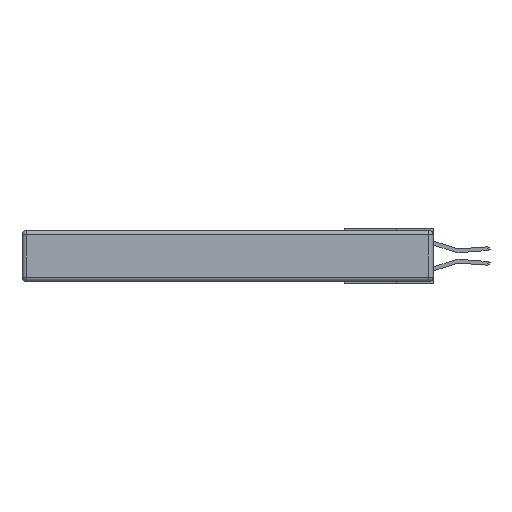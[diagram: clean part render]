
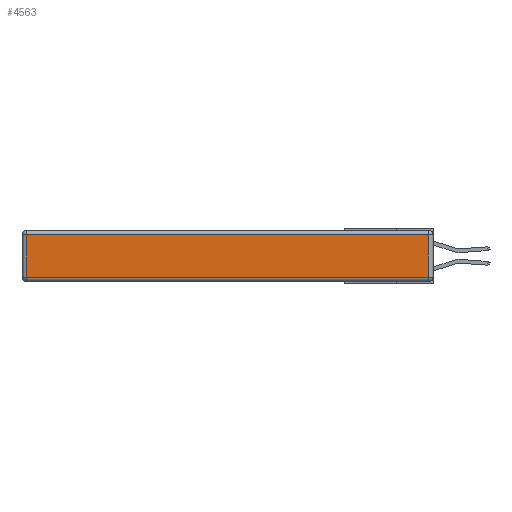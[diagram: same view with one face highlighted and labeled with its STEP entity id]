
A CAD part, left-side view. The second image highlights one B-rep face of the part: STEP entity #4563.
In plain terms, the highlighted planar face has unit normal (-1, 0, 0).
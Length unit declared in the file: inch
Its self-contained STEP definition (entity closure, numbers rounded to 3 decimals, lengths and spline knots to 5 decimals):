
#254 = EDGE_LOOP ( 'NONE', ( #12194, #11141, #3514, #7968 ) ) ;
#771 = CARTESIAN_POINT ( 'NONE',  ( 0., 0.03, -0.313 ) ) ;
#795 = VERTEX_POINT ( 'NONE', #9223 ) ;
#1589 = VECTOR ( 'NONE', #9602, 39.37008 ) ;
#1699 = DIRECTION ( 'NONE',  ( 0., 0., 1. ) ) ;
#2094 = VECTOR ( 'NONE', #2577, 39.37008 ) ;
#2219 = DIRECTION ( 'NONE',  ( 0., 0., 1. ) ) ;
#2357 = EDGE_CURVE ( 'NONE', #6201, #795, #15853, .T. ) ;
#2577 = DIRECTION ( 'NONE',  ( 0., -1., 0. ) ) ;
#3514 = ORIENTED_EDGE ( 'NONE', *, *, #5901, .T. ) ;
#4123 = CARTESIAN_POINT ( 'NONE',  ( 0., 0.03, -0.343 ) ) ;
#4563 = ADVANCED_FACE ( 'NONE', ( #13654 ), #7229, .T. ) ;
#4790 = VECTOR ( 'NONE', #1699, 39.37008 ) ;
#5390 = LINE ( 'NONE', #11068, #2094 ) ;
#5901 = EDGE_CURVE ( 'NONE', #795, #10869, #13213, .T. ) ;
#6201 = VERTEX_POINT ( 'NONE', #771 ) ;
#6334 = LINE ( 'NONE', #12099, #10789 ) ;
#6416 = DIRECTION ( 'NONE',  ( -1., 0., 0. ) ) ;
#7229 = PLANE ( 'NONE',  #9062 ) ;
#7968 = ORIENTED_EDGE ( 'NONE', *, *, #10000, .T. ) ;
#8332 = EDGE_CURVE ( 'NONE', #9868, #6201, #5390, .T. ) ;
#8535 = CARTESIAN_POINT ( 'NONE',  ( 0., 2.75, -0.03 ) ) ;
#9062 = AXIS2_PLACEMENT_3D ( 'NONE', #9787, #6416, #2219 ) ;
#9223 = CARTESIAN_POINT ( 'NONE',  ( 0., 0.03, -0.03 ) ) ;
#9602 = DIRECTION ( 'NONE',  ( 0., 1., 0. ) ) ;
#9787 = CARTESIAN_POINT ( 'NONE',  ( 0., 0., -0.343 ) ) ;
#9868 = VERTEX_POINT ( 'NONE', #14330 ) ;
#10000 = EDGE_CURVE ( 'NONE', #10869, #9868, #6334, .T. ) ;
#10789 = VECTOR ( 'NONE', #15687, 39.37008 ) ;
#10869 = VERTEX_POINT ( 'NONE', #11269 ) ;
#11068 = CARTESIAN_POINT ( 'NONE',  ( 0., 0., -0.313 ) ) ;
#11141 = ORIENTED_EDGE ( 'NONE', *, *, #2357, .T. ) ;
#11269 = CARTESIAN_POINT ( 'NONE',  ( 0., 2.72, -0.03 ) ) ;
#12099 = CARTESIAN_POINT ( 'NONE',  ( 0., 2.72, -0.343 ) ) ;
#12194 = ORIENTED_EDGE ( 'NONE', *, *, #8332, .T. ) ;
#13213 = LINE ( 'NONE', #8535, #1589 ) ;
#13654 = FACE_OUTER_BOUND ( 'NONE', #254, .T. ) ;
#14330 = CARTESIAN_POINT ( 'NONE',  ( 0., 2.72, -0.313 ) ) ;
#15687 = DIRECTION ( 'NONE',  ( 0., 0., -1. ) ) ;
#15853 = LINE ( 'NONE', #4123, #4790 ) ;
